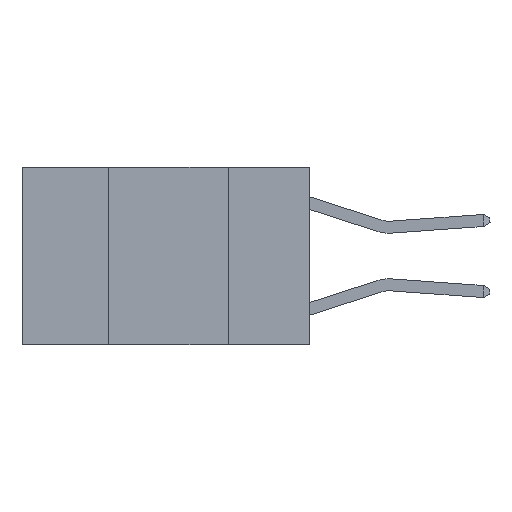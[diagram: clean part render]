
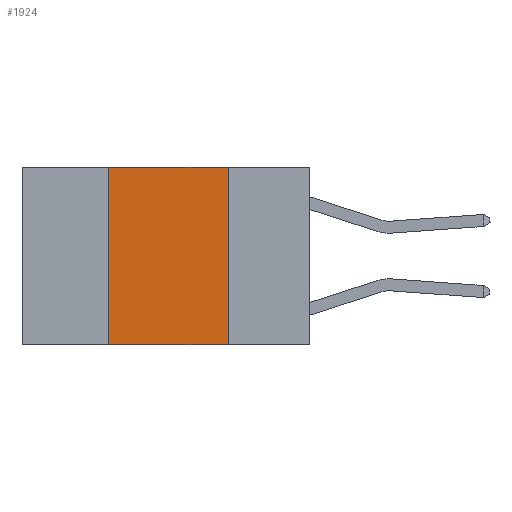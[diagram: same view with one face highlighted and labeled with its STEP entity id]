
A CAD part, left-side view. The second image highlights one B-rep face of the part: STEP entity #1924.
In plain terms, the highlighted planar face has unit normal (-1, 0, 0).
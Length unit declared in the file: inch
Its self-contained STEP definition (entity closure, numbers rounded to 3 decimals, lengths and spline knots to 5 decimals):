
#346 = CARTESIAN_POINT ( 'NONE',  ( 0., 0.6, 0. ) ) ;
#1565 = CARTESIAN_POINT ( 'NONE',  ( 0., 0.42, 0. ) ) ;
#1924 = ADVANCED_FACE ( 'NONE', ( #6480 ), #3415, .F. ) ;
#2094 = AXIS2_PLACEMENT_3D ( 'NONE', #8929, #13125, #4818 ) ;
#2552 = VERTEX_POINT ( 'NONE', #12929 ) ;
#2954 = CARTESIAN_POINT ( 'NONE',  ( 0., 0.17, 0. ) ) ;
#3000 = VECTOR ( 'NONE', #12683, 39.37008 ) ;
#3026 = VERTEX_POINT ( 'NONE', #9728 ) ;
#3415 = PLANE ( 'NONE',  #2094 ) ;
#4499 = DIRECTION ( 'NONE',  ( 0., 0., -1. ) ) ;
#4818 = DIRECTION ( 'NONE',  ( 0., 0., -1. ) ) ;
#5551 = VERTEX_POINT ( 'NONE', #2954 ) ;
#5609 = EDGE_CURVE ( 'NONE', #5551, #12633, #10643, .T. ) ;
#5777 = ORIENTED_EDGE ( 'NONE', *, *, #5609, .F. ) ;
#5816 = VECTOR ( 'NONE', #17650, 39.37008 ) ;
#6480 = FACE_OUTER_BOUND ( 'NONE', #11104, .T. ) ;
#7244 = EDGE_CURVE ( 'NONE', #2552, #3026, #8029, .T. ) ;
#7264 = CARTESIAN_POINT ( 'NONE',  ( 0., 0.17, -0.37 ) ) ;
#7476 = ORIENTED_EDGE ( 'NONE', *, *, #7244, .F. ) ;
#7973 = CARTESIAN_POINT ( 'NONE',  ( 0., 0.6, -0.37 ) ) ;
#8029 = LINE ( 'NONE', #1565, #3000 ) ;
#8459 = VECTOR ( 'NONE', #10027, 39.37008 ) ;
#8929 = CARTESIAN_POINT ( 'NONE',  ( 0., 0.6, 0. ) ) ;
#9309 = LINE ( 'NONE', #346, #8459 ) ;
#9404 = EDGE_CURVE ( 'NONE', #3026, #5551, #9309, .T. ) ;
#9728 = CARTESIAN_POINT ( 'NONE',  ( 0., 0.42, 0. ) ) ;
#10027 = DIRECTION ( 'NONE',  ( 0., -1., 0. ) ) ;
#10643 = LINE ( 'NONE', #12796, #14361 ) ;
#11104 = EDGE_LOOP ( 'NONE', ( #5777, #17274, #7476, #17918 ) ) ;
#12633 = VERTEX_POINT ( 'NONE', #7264 ) ;
#12683 = DIRECTION ( 'NONE',  ( 0., 0., 1. ) ) ;
#12796 = CARTESIAN_POINT ( 'NONE',  ( 0., 0.17, 0. ) ) ;
#12929 = CARTESIAN_POINT ( 'NONE',  ( 0., 0.42, -0.37 ) ) ;
#13125 = DIRECTION ( 'NONE',  ( 1., 0., 0. ) ) ;
#14361 = VECTOR ( 'NONE', #4499, 39.37008 ) ;
#15910 = EDGE_CURVE ( 'NONE', #2552, #12633, #16839, .T. ) ;
#16839 = LINE ( 'NONE', #7973, #5816 ) ;
#17274 = ORIENTED_EDGE ( 'NONE', *, *, #9404, .F. ) ;
#17650 = DIRECTION ( 'NONE',  ( 0., -1., 0. ) ) ;
#17918 = ORIENTED_EDGE ( 'NONE', *, *, #15910, .T. ) ;
